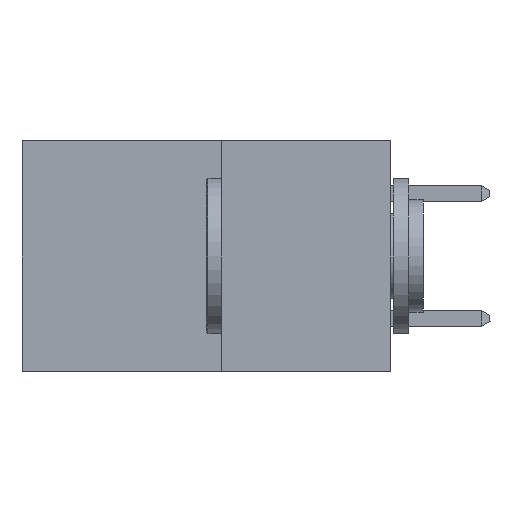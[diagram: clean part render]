
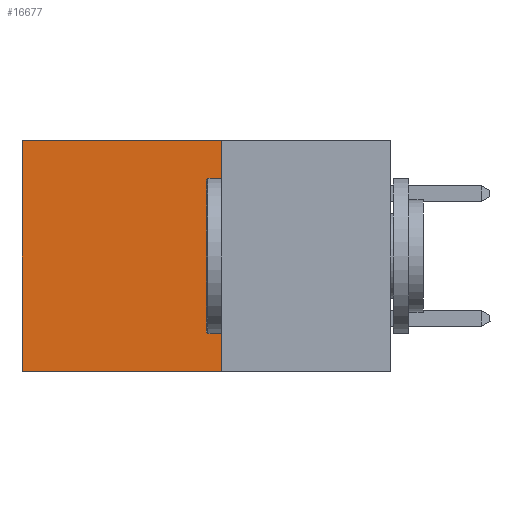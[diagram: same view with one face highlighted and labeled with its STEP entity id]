
A CAD part, left-side view. The second image highlights one B-rep face of the part: STEP entity #16677.
In plain terms, the highlighted planar face has unit normal (-1, 0, 0).
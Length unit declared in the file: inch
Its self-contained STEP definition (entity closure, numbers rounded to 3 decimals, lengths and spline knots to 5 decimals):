
#1296 = VECTOR ( 'NONE', #15387, 39.37008 ) ;
#1473 = CARTESIAN_POINT ( 'NONE',  ( 0.277, 0.27, -0.37 ) ) ;
#2031 = CARTESIAN_POINT ( 'NONE',  ( 0.277, 0.27, -0.37 ) ) ;
#2147 = LINE ( 'NONE', #12996, #20002 ) ;
#3730 = EDGE_CURVE ( 'NONE', #20007, #18664, #3913, .T. ) ;
#3758 = EDGE_LOOP ( 'NONE', ( #8183, #17718, #17803, #9487 ) ) ;
#3838 = DIRECTION ( 'NONE',  ( 0., 0., -1. ) ) ;
#3913 = LINE ( 'NONE', #16687, #21658 ) ;
#4026 = VERTEX_POINT ( 'NONE', #15602 ) ;
#5380 = CARTESIAN_POINT ( 'NONE',  ( 0.277, 0.27, 0. ) ) ;
#5678 = EDGE_CURVE ( 'NONE', #4026, #18664, #2147, .T. ) ;
#6031 = VECTOR ( 'NONE', #18530, 39.37008 ) ;
#6579 = CARTESIAN_POINT ( 'NONE',  ( 0.277, 0.27, 0. ) ) ;
#7908 = AXIS2_PLACEMENT_3D ( 'NONE', #2031, #14168, #3838 ) ;
#8183 = ORIENTED_EDGE ( 'NONE', *, *, #3730, .T. ) ;
#8773 = CARTESIAN_POINT ( 'NONE',  ( 0.277, 0.59, -0.37 ) ) ;
#9487 = ORIENTED_EDGE ( 'NONE', *, *, #22322, .T. ) ;
#12463 = PLANE ( 'NONE',  #7908 ) ;
#12602 = DIRECTION ( 'NONE',  ( 0., 1., 0. ) ) ;
#12996 = CARTESIAN_POINT ( 'NONE',  ( 0.277, 0.27, -0.37 ) ) ;
#13741 = VERTEX_POINT ( 'NONE', #5380 ) ;
#14168 = DIRECTION ( 'NONE',  ( 1., 0., 0. ) ) ;
#15223 = CARTESIAN_POINT ( 'NONE',  ( 0.277, 0.59, 0. ) ) ;
#15387 = DIRECTION ( 'NONE',  ( 0., 0., -1. ) ) ;
#15576 = DIRECTION ( 'NONE',  ( 0., 0., -1. ) ) ;
#15602 = CARTESIAN_POINT ( 'NONE',  ( 0.277, 0.27, -0.37 ) ) ;
#15715 = EDGE_CURVE ( 'NONE', #13741, #4026, #15726, .T. ) ;
#15726 = LINE ( 'NONE', #1473, #1296 ) ;
#16677 = ADVANCED_FACE ( 'NONE', ( #18092 ), #12463, .F. ) ;
#16687 = CARTESIAN_POINT ( 'NONE',  ( 0.277, 0.59, -0.37 ) ) ;
#17718 = ORIENTED_EDGE ( 'NONE', *, *, #5678, .F. ) ;
#17803 = ORIENTED_EDGE ( 'NONE', *, *, #15715, .F. ) ;
#18092 = FACE_OUTER_BOUND ( 'NONE', #3758, .T. ) ;
#18530 = DIRECTION ( 'NONE',  ( 0., 1., 0. ) ) ;
#18664 = VERTEX_POINT ( 'NONE', #8773 ) ;
#19698 = LINE ( 'NONE', #6579, #6031 ) ;
#20002 = VECTOR ( 'NONE', #12602, 39.37008 ) ;
#20007 = VERTEX_POINT ( 'NONE', #15223 ) ;
#21658 = VECTOR ( 'NONE', #15576, 39.37008 ) ;
#22322 = EDGE_CURVE ( 'NONE', #13741, #20007, #19698, .T. ) ;
